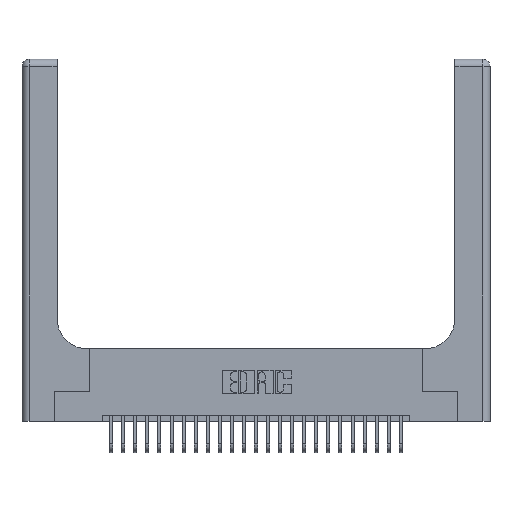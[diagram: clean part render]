
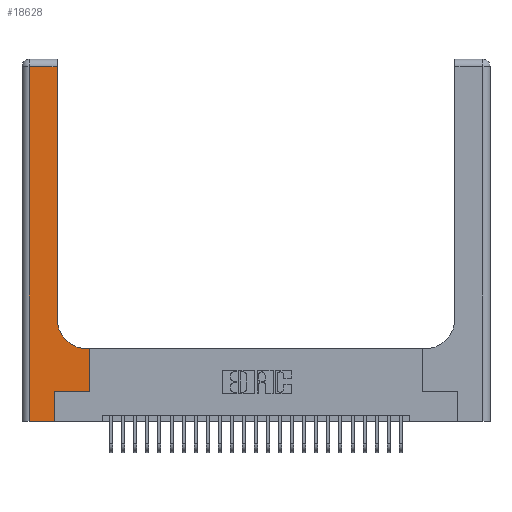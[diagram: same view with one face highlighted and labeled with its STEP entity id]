
A CAD part, top view. The second image highlights one B-rep face of the part: STEP entity #18628.
In plain terms, the highlighted planar face has unit normal (0, 0, 1).
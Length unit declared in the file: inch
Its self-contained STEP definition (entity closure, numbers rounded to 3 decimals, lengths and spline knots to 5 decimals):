
#434 = VERTEX_POINT ( 'NONE', #14833 ) ;
#1824 = ORIENTED_EDGE ( 'NONE', *, *, #20376, .T. ) ;
#1871 = VERTEX_POINT ( 'NONE', #27894 ) ;
#2066 = LINE ( 'NONE', #10234, #13178 ) ;
#2094 = EDGE_CURVE ( 'NONE', #18840, #14676, #15600, .T. ) ;
#2540 = DIRECTION ( 'NONE',  ( 0., 1., 0. ) ) ;
#2866 = DIRECTION ( 'NONE',  ( 0., 0., -1. ) ) ;
#2895 = DIRECTION ( 'NONE',  ( 0., 0., -1. ) ) ;
#3597 = VECTOR ( 'NONE', #18729, 39.37008 ) ;
#4075 = CARTESIAN_POINT ( 'NONE',  ( 0., 0., 0.37 ) ) ;
#4171 = ORIENTED_EDGE ( 'NONE', *, *, #2094, .T. ) ;
#4818 = VERTEX_POINT ( 'NONE', #9843 ) ;
#5132 = ORIENTED_EDGE ( 'NONE', *, *, #18031, .T. ) ;
#5139 = DIRECTION ( 'NONE',  ( -1., 0., 0. ) ) ;
#5199 = ORIENTED_EDGE ( 'NONE', *, *, #14738, .T. ) ;
#5785 = EDGE_CURVE ( 'NONE', #6119, #11556, #2066, .T. ) ;
#6119 = VERTEX_POINT ( 'NONE', #24310 ) ;
#6222 = ORIENTED_EDGE ( 'NONE', *, *, #20094, .T. ) ;
#7766 = CARTESIAN_POINT ( 'NONE',  ( 0.2915, 0.85, 0.37 ) ) ;
#8502 = DIRECTION ( 'NONE',  ( -1., 0., 0. ) ) ;
#8898 = LINE ( 'NONE', #15763, #22769 ) ;
#9843 = CARTESIAN_POINT ( 'NONE',  ( 0.5585, 0.25, 0.37 ) ) ;
#10234 = CARTESIAN_POINT ( 'NONE',  ( 0.2915, 0.6, 0.37 ) ) ;
#10538 = CARTESIAN_POINT ( 'NONE',  ( 0.2915, 2.94, 0.37 ) ) ;
#10677 = DIRECTION ( 'NONE',  ( 1., 0., 0. ) ) ;
#11244 = EDGE_CURVE ( 'NONE', #434, #4818, #24253, .T. ) ;
#11365 = CARTESIAN_POINT ( 'NONE',  ( 0.06, 0., 0.37 ) ) ;
#11493 = LINE ( 'NONE', #4075, #20474 ) ;
#11556 = VERTEX_POINT ( 'NONE', #19635 ) ;
#12689 = VERTEX_POINT ( 'NONE', #19014 ) ;
#13178 = VECTOR ( 'NONE', #8502, 39.37008 ) ;
#13437 = EDGE_CURVE ( 'NONE', #14676, #1871, #17167, .T. ) ;
#13525 = ORIENTED_EDGE ( 'NONE', *, *, #5785, .T. ) ;
#13588 = CARTESIAN_POINT ( 'NONE',  ( 0.06, 3., 0.37 ) ) ;
#14164 = DIRECTION ( 'NONE',  ( 1., 0., 0. ) ) ;
#14470 = ORIENTED_EDGE ( 'NONE', *, *, #11244, .T. ) ;
#14676 = VERTEX_POINT ( 'NONE', #10538 ) ;
#14738 = EDGE_CURVE ( 'NONE', #12689, #434, #24770, .T. ) ;
#14833 = CARTESIAN_POINT ( 'NONE',  ( 0.269, 0.25, 0.37 ) ) ;
#15600 = LINE ( 'NONE', #28043, #23583 ) ;
#15763 = CARTESIAN_POINT ( 'NONE',  ( 0.5585, 0.25, 0.37 ) ) ;
#16208 = CARTESIAN_POINT ( 'NONE',  ( 0.5415, 0.85, 0.37 ) ) ;
#16277 = AXIS2_PLACEMENT_3D ( 'NONE', #16208, #2895, #14164 ) ;
#16588 = EDGE_CURVE ( 'NONE', #4818, #6119, #8898, .T. ) ;
#16802 = LINE ( 'NONE', #13588, #3597 ) ;
#16804 = DIRECTION ( 'NONE',  ( 1., 0., 0. ) ) ;
#17167 = LINE ( 'NONE', #20138, #19939 ) ;
#18031 = EDGE_CURVE ( 'NONE', #1871, #26517, #16802, .T. ) ;
#18270 = DIRECTION ( 'NONE',  ( 0., 1., 0. ) ) ;
#18406 = CARTESIAN_POINT ( 'NONE',  ( 0., 3., 0.37 ) ) ;
#18628 = ADVANCED_FACE ( 'NONE', ( #22328 ), #25004, .F. ) ;
#18729 = DIRECTION ( 'NONE',  ( 0., -1., 0. ) ) ;
#18738 = ORIENTED_EDGE ( 'NONE', *, *, #16588, .T. ) ;
#18840 = VERTEX_POINT ( 'NONE', #7766 ) ;
#19014 = CARTESIAN_POINT ( 'NONE',  ( 0.269, 0., 0.37 ) ) ;
#19415 = AXIS2_PLACEMENT_3D ( 'NONE', #18406, #2866, #5139 ) ;
#19635 = CARTESIAN_POINT ( 'NONE',  ( 0.5415, 0.6, 0.37 ) ) ;
#19939 = VECTOR ( 'NONE', #24806, 39.37008 ) ;
#20094 = EDGE_CURVE ( 'NONE', #11556, #18840, #23642, .T. ) ;
#20138 = CARTESIAN_POINT ( 'NONE',  ( 0., 2.94, 0.37 ) ) ;
#20284 = CARTESIAN_POINT ( 'NONE',  ( 0.269, 0., 0.37 ) ) ;
#20376 = EDGE_CURVE ( 'NONE', #26517, #12689, #11493, .T. ) ;
#20474 = VECTOR ( 'NONE', #10677, 39.37008 ) ;
#22328 = FACE_OUTER_BOUND ( 'NONE', #28594, .T. ) ;
#22769 = VECTOR ( 'NONE', #18270, 39.37008 ) ;
#23583 = VECTOR ( 'NONE', #25785, 39.37008 ) ;
#23642 = CIRCLE ( 'NONE', #16277, 0.25 ) ;
#24253 = LINE ( 'NONE', #25449, #24928 ) ;
#24310 = CARTESIAN_POINT ( 'NONE',  ( 0.5585, 0.6, 0.37 ) ) ;
#24770 = LINE ( 'NONE', #20284, #26202 ) ;
#24806 = DIRECTION ( 'NONE',  ( -1., 0., 0. ) ) ;
#24928 = VECTOR ( 'NONE', #16804, 39.37008 ) ;
#25004 = PLANE ( 'NONE',  #19415 ) ;
#25449 = CARTESIAN_POINT ( 'NONE',  ( 0.269, 0.25, 0.37 ) ) ;
#25785 = DIRECTION ( 'NONE',  ( 0., 1., 0. ) ) ;
#26134 = ORIENTED_EDGE ( 'NONE', *, *, #13437, .T. ) ;
#26202 = VECTOR ( 'NONE', #2540, 39.37008 ) ;
#26517 = VERTEX_POINT ( 'NONE', #11365 ) ;
#27894 = CARTESIAN_POINT ( 'NONE',  ( 0.06, 2.94, 0.37 ) ) ;
#28043 = CARTESIAN_POINT ( 'NONE',  ( 0.2915, 3., 0.37 ) ) ;
#28594 = EDGE_LOOP ( 'NONE', ( #4171, #26134, #5132, #1824, #5199, #14470, #18738, #13525, #6222 ) ) ;
